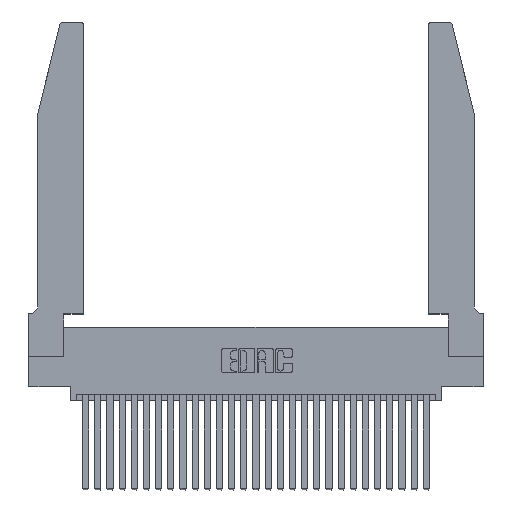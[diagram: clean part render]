
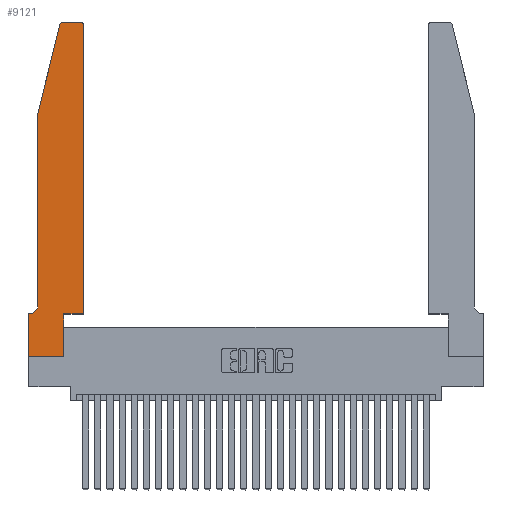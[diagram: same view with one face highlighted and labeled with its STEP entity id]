
A CAD part, top view. The second image highlights one B-rep face of the part: STEP entity #9121.
In plain terms, the highlighted planar face has unit normal (0, 0, 1).
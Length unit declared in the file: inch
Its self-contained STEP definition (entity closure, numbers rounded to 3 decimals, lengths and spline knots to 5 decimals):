
#248 = VERTEX_POINT ( 'NONE', #10417 ) ;
#264 = CIRCLE ( 'NONE', #15518, 0.03 ) ;
#349 = EDGE_CURVE ( 'NONE', #18495, #2752, #8665, .T. ) ;
#413 = LINE ( 'NONE', #6374, #23856 ) ;
#533 = CARTESIAN_POINT ( 'NONE',  ( 0.4505, 2.72, 0.37 ) ) ;
#738 = ORIENTED_EDGE ( 'NONE', *, *, #17567, .T. ) ;
#999 = CARTESIAN_POINT ( 'NONE',  ( 0., 0.35, 0.37 ) ) ;
#1176 = DIRECTION ( 'NONE',  ( 1., 0., 0. ) ) ;
#1266 = VERTEX_POINT ( 'NONE', #26140 ) ;
#1370 = LINE ( 'NONE', #2965, #18807 ) ;
#1381 = AXIS2_PLACEMENT_3D ( 'NONE', #7194, #22996, #9516 ) ;
#1611 = VERTEX_POINT ( 'NONE', #533 ) ;
#1909 = EDGE_CURVE ( 'NONE', #13605, #14582, #1370, .T. ) ;
#2285 = FACE_OUTER_BOUND ( 'NONE', #2950, .T. ) ;
#2752 = VERTEX_POINT ( 'NONE', #15708 ) ;
#2950 = EDGE_LOOP ( 'NONE', ( #25375, #15954, #19876, #7207, #20987, #8627, #10170, #738, #14040, #22302, #15532, #22809 ) ) ;
#2965 = CARTESIAN_POINT ( 'NONE',  ( 0., 0., 0.37 ) ) ;
#3322 = PLANE ( 'NONE',  #7305 ) ;
#3658 = EDGE_CURVE ( 'NONE', #22092, #15027, #5241, .T. ) ;
#3930 = VECTOR ( 'NONE', #15695, 39.37008 ) ;
#4162 = CARTESIAN_POINT ( 'NONE',  ( 0.0755, 0.35, 0.37 ) ) ;
#4441 = DIRECTION ( 'NONE',  ( -1., 0., 0. ) ) ;
#4476 = CIRCLE ( 'NONE', #27768, 0.07 ) ;
#5041 = LINE ( 'NONE', #21651, #16437 ) ;
#5241 = LINE ( 'NONE', #14875, #12379 ) ;
#6018 = CARTESIAN_POINT ( 'NONE',  ( 0.284, 2.72, 0.37 ) ) ;
#6374 = CARTESIAN_POINT ( 'NONE',  ( 0.4505, 0.35, 0.37 ) ) ;
#7194 = CARTESIAN_POINT ( 'NONE',  ( 0.4205, 2.72, 0.37 ) ) ;
#7207 = ORIENTED_EDGE ( 'NONE', *, *, #23100, .T. ) ;
#7305 = AXIS2_PLACEMENT_3D ( 'NONE', #999, #21475, #7954 ) ;
#7954 = DIRECTION ( 'NONE',  ( 1., 0., 0. ) ) ;
#8099 = CARTESIAN_POINT ( 'NONE',  ( 0.0055, 0.42, 0.37 ) ) ;
#8188 = CARTESIAN_POINT ( 'NONE',  ( 0., 0., 0.37 ) ) ;
#8366 = DIRECTION ( 'NONE',  ( 1., 0., 0. ) ) ;
#8464 = CARTESIAN_POINT ( 'NONE',  ( 0.0055, 0.35, 0.37 ) ) ;
#8585 = VERTEX_POINT ( 'NONE', #9253 ) ;
#8627 = ORIENTED_EDGE ( 'NONE', *, *, #12316, .T. ) ;
#8665 = LINE ( 'NONE', #14686, #14703 ) ;
#8704 = DIRECTION ( 'NONE',  ( 0., 1., 0. ) ) ;
#9121 = ADVANCED_FACE ( 'NONE', ( #2285 ), #3322, .T. ) ;
#9253 = CARTESIAN_POINT ( 'NONE',  ( 0.0755, 0.42, 0.37 ) ) ;
#9516 = DIRECTION ( 'NONE',  ( 1., 0., 0. ) ) ;
#9927 = EDGE_CURVE ( 'NONE', #15027, #1611, #413, .T. ) ;
#10170 = ORIENTED_EDGE ( 'NONE', *, *, #1909, .T. ) ;
#10404 = DIRECTION ( 'NONE',  ( -1., 0., 0. ) ) ;
#10417 = CARTESIAN_POINT ( 'NONE',  ( 0.284, 2.75, 0.37 ) ) ;
#10757 = CIRCLE ( 'NONE', #1381, 0.03 ) ;
#11446 = EDGE_CURVE ( 'NONE', #1611, #1266, #10757, .T. ) ;
#12301 = CARTESIAN_POINT ( 'NONE',  ( 0.2865, 0.35, 0.37 ) ) ;
#12316 = EDGE_CURVE ( 'NONE', #28484, #13605, #25482, .T. ) ;
#12379 = VECTOR ( 'NONE', #1176, 39.37008 ) ;
#12688 = LINE ( 'NONE', #24798, #17965 ) ;
#13605 = VERTEX_POINT ( 'NONE', #26874 ) ;
#14040 = ORIENTED_EDGE ( 'NONE', *, *, #27778, .T. ) ;
#14582 = VERTEX_POINT ( 'NONE', #8188 ) ;
#14686 = CARTESIAN_POINT ( 'NONE',  ( 0.0755, 2., 0.37 ) ) ;
#14703 = VECTOR ( 'NONE', #19485, 39.37008 ) ;
#14875 = CARTESIAN_POINT ( 'NONE',  ( 0.4505, 0.35, 0.37 ) ) ;
#15027 = VERTEX_POINT ( 'NONE', #27855 ) ;
#15518 = AXIS2_PLACEMENT_3D ( 'NONE', #6018, #21887, #8366 ) ;
#15532 = ORIENTED_EDGE ( 'NONE', *, *, #9927, .T. ) ;
#15612 = DIRECTION ( 'NONE',  ( -1., 0., 0. ) ) ;
#15695 = DIRECTION ( 'NONE',  ( 0., -1., 0. ) ) ;
#15708 = CARTESIAN_POINT ( 'NONE',  ( 0.0755, 2., 0.37 ) ) ;
#15954 = ORIENTED_EDGE ( 'NONE', *, *, #24455, .T. ) ;
#16437 = VECTOR ( 'NONE', #23862, 39.37008 ) ;
#16652 = CARTESIAN_POINT ( 'NONE',  ( 0.25487, 2.72718, 0.37 ) ) ;
#17567 = EDGE_CURVE ( 'NONE', #14582, #27418, #21403, .T. ) ;
#17965 = VECTOR ( 'NONE', #4441, 39.37008 ) ;
#18495 = VERTEX_POINT ( 'NONE', #16652 ) ;
#18807 = VECTOR ( 'NONE', #20520, 39.37008 ) ;
#18842 = VECTOR ( 'NONE', #15612, 39.37008 ) ;
#19485 = DIRECTION ( 'NONE',  ( -0.239, -0.971, 0. ) ) ;
#19637 = EDGE_CURVE ( 'NONE', #8585, #28484, #4476, .T. ) ;
#19876 = ORIENTED_EDGE ( 'NONE', *, *, #349, .T. ) ;
#20520 = DIRECTION ( 'NONE',  ( 0., -1., 0. ) ) ;
#20678 = VECTOR ( 'NONE', #25339, 39.37008 ) ;
#20987 = ORIENTED_EDGE ( 'NONE', *, *, #19637, .T. ) ;
#21321 = LINE ( 'NONE', #28999, #3930 ) ;
#21403 = LINE ( 'NONE', #23102, #20678 ) ;
#21475 = DIRECTION ( 'NONE',  ( 0., 0., 1. ) ) ;
#21651 = CARTESIAN_POINT ( 'NONE',  ( 0.2865, 0.35, 0.37 ) ) ;
#21887 = DIRECTION ( 'NONE',  ( 0., 0., 1. ) ) ;
#22092 = VERTEX_POINT ( 'NONE', #12301 ) ;
#22302 = ORIENTED_EDGE ( 'NONE', *, *, #3658, .T. ) ;
#22809 = ORIENTED_EDGE ( 'NONE', *, *, #11446, .T. ) ;
#22996 = DIRECTION ( 'NONE',  ( 0., 0., 1. ) ) ;
#23100 = EDGE_CURVE ( 'NONE', #2752, #8585, #21321, .T. ) ;
#23102 = CARTESIAN_POINT ( 'NONE',  ( 0., 0., 0.37 ) ) ;
#23846 = DIRECTION ( 'NONE',  ( 0., 0., -1. ) ) ;
#23856 = VECTOR ( 'NONE', #8704, 39.37008 ) ;
#23862 = DIRECTION ( 'NONE',  ( 0., 1., 0. ) ) ;
#24455 = EDGE_CURVE ( 'NONE', #248, #18495, #264, .T. ) ;
#24798 = CARTESIAN_POINT ( 'NONE',  ( 0.2605, 2.75, 0.37 ) ) ;
#25339 = DIRECTION ( 'NONE',  ( 1., 0., 0. ) ) ;
#25375 = ORIENTED_EDGE ( 'NONE', *, *, #25944, .T. ) ;
#25482 = LINE ( 'NONE', #4162, #18842 ) ;
#25944 = EDGE_CURVE ( 'NONE', #1266, #248, #12688, .T. ) ;
#26140 = CARTESIAN_POINT ( 'NONE',  ( 0.4205, 2.75, 0.37 ) ) ;
#26874 = CARTESIAN_POINT ( 'NONE',  ( 0., 0.35, 0.37 ) ) ;
#26876 = CARTESIAN_POINT ( 'NONE',  ( 0.2865, 0., 0.37 ) ) ;
#27418 = VERTEX_POINT ( 'NONE', #26876 ) ;
#27768 = AXIS2_PLACEMENT_3D ( 'NONE', #8099, #23846, #10404 ) ;
#27778 = EDGE_CURVE ( 'NONE', #27418, #22092, #5041, .T. ) ;
#27855 = CARTESIAN_POINT ( 'NONE',  ( 0.4505, 0.35, 0.37 ) ) ;
#28484 = VERTEX_POINT ( 'NONE', #8464 ) ;
#28999 = CARTESIAN_POINT ( 'NONE',  ( 0.0755, 2., 0.37 ) ) ;
